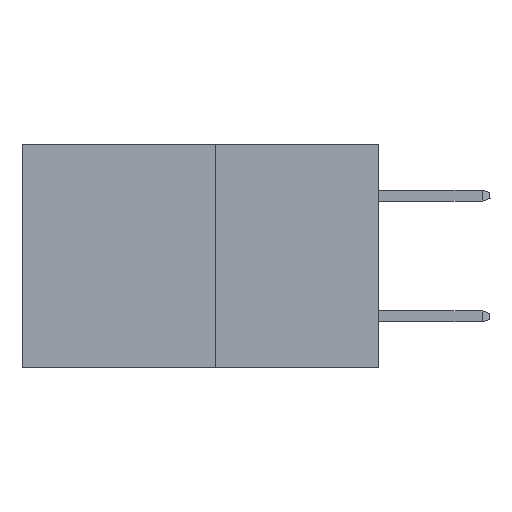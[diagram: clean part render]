
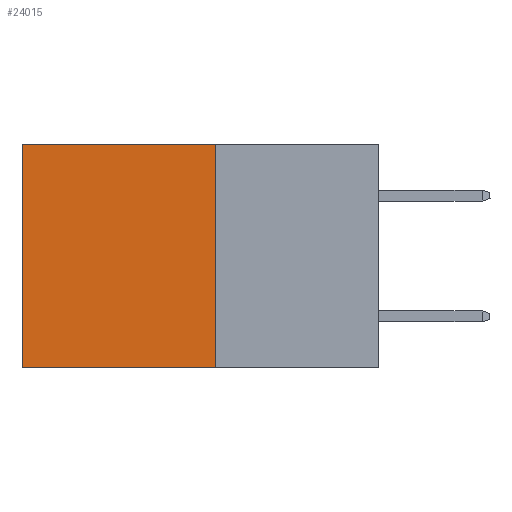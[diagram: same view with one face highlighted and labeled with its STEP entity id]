
A CAD part, left-side view. The second image highlights one B-rep face of the part: STEP entity #24015.
In plain terms, the highlighted planar face has unit normal (-1, 0, 0).
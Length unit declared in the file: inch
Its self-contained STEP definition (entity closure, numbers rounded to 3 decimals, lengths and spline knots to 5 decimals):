
#182 = CARTESIAN_POINT ( 'NONE',  ( 0.277, 0.27, -0.37 ) ) ;
#266 = DIRECTION ( 'NONE',  ( 0., 0., -1. ) ) ;
#1064 = CARTESIAN_POINT ( 'NONE',  ( 0.277, 0.59, 0. ) ) ;
#2074 = CARTESIAN_POINT ( 'NONE',  ( 0.277, 0.27, 0. ) ) ;
#3520 = EDGE_CURVE ( 'NONE', #22233, #12620, #13879, .T. ) ;
#3566 = DIRECTION ( 'NONE',  ( 0., 1., 0. ) ) ;
#3611 = EDGE_CURVE ( 'NONE', #12620, #13635, #22618, .T. ) ;
#3976 = AXIS2_PLACEMENT_3D ( 'NONE', #6448, #8507, #22576 ) ;
#4482 = ORIENTED_EDGE ( 'NONE', *, *, #3520, .F. ) ;
#4768 = ORIENTED_EDGE ( 'NONE', *, *, #12501, .T. ) ;
#5994 = CARTESIAN_POINT ( 'NONE',  ( 0.277, 0.27, -0.37 ) ) ;
#6448 = CARTESIAN_POINT ( 'NONE',  ( 0.277, 0.27, -0.37 ) ) ;
#6498 = ORIENTED_EDGE ( 'NONE', *, *, #20975, .T. ) ;
#6717 = CARTESIAN_POINT ( 'NONE',  ( 0.277, 0.59, -0.37 ) ) ;
#8507 = DIRECTION ( 'NONE',  ( 1., 0., 0. ) ) ;
#10727 = CARTESIAN_POINT ( 'NONE',  ( 0.277, 0.59, -0.37 ) ) ;
#10743 = EDGE_LOOP ( 'NONE', ( #6498, #24642, #4482, #4768 ) ) ;
#11320 = VECTOR ( 'NONE', #18105, 39.37008 ) ;
#12501 = EDGE_CURVE ( 'NONE', #22233, #25798, #20144, .T. ) ;
#12620 = VERTEX_POINT ( 'NONE', #5994 ) ;
#13635 = VERTEX_POINT ( 'NONE', #6717 ) ;
#13769 = CARTESIAN_POINT ( 'NONE',  ( 0.277, 0.27, 0. ) ) ;
#13879 = LINE ( 'NONE', #182, #24479 ) ;
#18105 = DIRECTION ( 'NONE',  ( 0., 1., 0. ) ) ;
#18520 = VECTOR ( 'NONE', #20856, 39.37008 ) ;
#18624 = PLANE ( 'NONE',  #3976 ) ;
#20100 = CARTESIAN_POINT ( 'NONE',  ( 0.277, 0.27, -0.37 ) ) ;
#20144 = LINE ( 'NONE', #13769, #25390 ) ;
#20856 = DIRECTION ( 'NONE',  ( 0., 0., -1. ) ) ;
#20975 = EDGE_CURVE ( 'NONE', #25798, #13635, #23748, .T. ) ;
#22233 = VERTEX_POINT ( 'NONE', #2074 ) ;
#22576 = DIRECTION ( 'NONE',  ( 0., 0., -1. ) ) ;
#22618 = LINE ( 'NONE', #20100, #11320 ) ;
#23748 = LINE ( 'NONE', #10727, #18520 ) ;
#24015 = ADVANCED_FACE ( 'NONE', ( #24568 ), #18624, .F. ) ;
#24479 = VECTOR ( 'NONE', #266, 39.37008 ) ;
#24568 = FACE_OUTER_BOUND ( 'NONE', #10743, .T. ) ;
#24642 = ORIENTED_EDGE ( 'NONE', *, *, #3611, .F. ) ;
#25390 = VECTOR ( 'NONE', #3566, 39.37008 ) ;
#25798 = VERTEX_POINT ( 'NONE', #1064 ) ;
